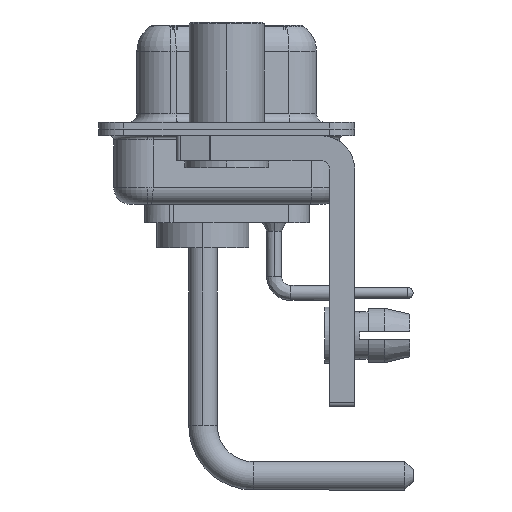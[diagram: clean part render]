
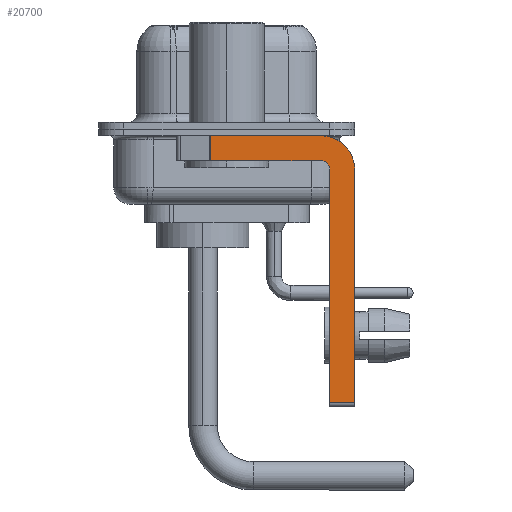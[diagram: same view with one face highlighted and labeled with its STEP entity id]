
A CAD part, left-side view. The second image highlights one B-rep face of the part: STEP entity #20700.
In plain terms, the highlighted planar face has unit normal (-1, 0, 0).
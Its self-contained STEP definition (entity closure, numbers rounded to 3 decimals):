
#186 = ORIENTED_EDGE ( 'NONE', *, *, #3425, .T. ) ;
#244 = VERTEX_POINT ( 'NONE', #5810 ) ;
#465 = VERTEX_POINT ( 'NONE', #19800 ) ;
#865 = LINE ( 'NONE', #9056, #3187 ) ;
#1306 = CARTESIAN_POINT ( 'NONE',  ( -2.9, -7.65, -2.4 ) ) ;
#1475 = CARTESIAN_POINT ( 'NONE',  ( -2.9, -5.65, -1.9 ) ) ;
#1550 = CARTESIAN_POINT ( 'NONE',  ( -2.9, -5.65, -1.9 ) ) ;
#1585 = AXIS2_PLACEMENT_3D ( 'NONE', #14145, #19778, #5796 ) ;
#1622 = DIRECTION ( 'NONE',  ( 1., 0., 0. ) ) ;
#2145 = VECTOR ( 'NONE', #5016, 1000. ) ;
#2606 = CARTESIAN_POINT ( 'NONE',  ( -2.9, -5.65, -2.4 ) ) ;
#2700 = LINE ( 'NONE', #22467, #2145 ) ;
#2841 = EDGE_CURVE ( 'NONE', #244, #4026, #12103, .T. ) ;
#2920 = CARTESIAN_POINT ( 'NONE',  ( -2.9, 3., -0.4 ) ) ;
#3058 = CARTESIAN_POINT ( 'NONE',  ( -2.9, -7.65, -2.4 ) ) ;
#3187 = VECTOR ( 'NONE', #5215, 1000. ) ;
#3425 = EDGE_CURVE ( 'NONE', #14927, #16375, #865, .T. ) ;
#4026 = VERTEX_POINT ( 'NONE', #23267 ) ;
#4551 = CARTESIAN_POINT ( 'NONE',  ( -2.9, -6.15, -2.4 ) ) ;
#5016 = DIRECTION ( 'NONE',  ( 0., 0., 1. ) ) ;
#5215 = DIRECTION ( 'NONE',  ( 0., 0., -1. ) ) ;
#5321 = VECTOR ( 'NONE', #22303, 1000. ) ;
#5400 = DIRECTION ( 'NONE',  ( 0., 0., -1. ) ) ;
#5796 = DIRECTION ( 'NONE',  ( 0., 0., 1. ) ) ;
#5810 = CARTESIAN_POINT ( 'NONE',  ( -2.9, -6.15, -16.35 ) ) ;
#6831 = ORIENTED_EDGE ( 'NONE', *, *, #7423, .F. ) ;
#6863 = ORIENTED_EDGE ( 'NONE', *, *, #2841, .T. ) ;
#6867 = VECTOR ( 'NONE', #23519, 1000. ) ;
#7423 = EDGE_CURVE ( 'NONE', #18078, #16375, #23031, .T. ) ;
#7521 = FACE_OUTER_BOUND ( 'NONE', #20593, .T. ) ;
#7648 = DIRECTION ( 'NONE',  ( 0., 0., -1. ) ) ;
#8011 = DIRECTION ( 'NONE',  ( 1., 0., 0. ) ) ;
#8805 = VECTOR ( 'NONE', #19782, 1000. ) ;
#9056 = CARTESIAN_POINT ( 'NONE',  ( -2.9, 0.978, -1.9 ) ) ;
#9861 = AXIS2_PLACEMENT_3D ( 'NONE', #13315, #1622, #7648 ) ;
#10473 = ORIENTED_EDGE ( 'NONE', *, *, #22078, .F. ) ;
#12103 = LINE ( 'NONE', #16083, #6867 ) ;
#12815 = ORIENTED_EDGE ( 'NONE', *, *, #14926, .F. ) ;
#13247 = LINE ( 'NONE', #1306, #14360 ) ;
#13315 = CARTESIAN_POINT ( 'NONE',  ( -2.9, -5.65, -2.4 ) ) ;
#13697 = ORIENTED_EDGE ( 'NONE', *, *, #19569, .F. ) ;
#14145 = CARTESIAN_POINT ( 'NONE',  ( -2.9, -5.65, -2.4 ) ) ;
#14195 = EDGE_CURVE ( 'NONE', #17536, #18078, #14717, .T. ) ;
#14360 = VECTOR ( 'NONE', #5400, 1000. ) ;
#14717 = CIRCLE ( 'NONE', #1585, 0.5 ) ;
#14926 = EDGE_CURVE ( 'NONE', #14927, #465, #20127, .T. ) ;
#14927 = VERTEX_POINT ( 'NONE', #18211 ) ;
#15280 = ORIENTED_EDGE ( 'NONE', *, *, #22847, .F. ) ;
#16083 = CARTESIAN_POINT ( 'NONE',  ( -2.9, -5.65, -16.35 ) ) ;
#16231 = DIRECTION ( 'NONE',  ( 0., 0., -1. ) ) ;
#16375 = VERTEX_POINT ( 'NONE', #18848 ) ;
#16972 = CIRCLE ( 'NONE', #23502, 2. ) ;
#17536 = VERTEX_POINT ( 'NONE', #4551 ) ;
#18078 = VERTEX_POINT ( 'NONE', #1550 ) ;
#18211 = CARTESIAN_POINT ( 'NONE',  ( -2.9, 0.978, -0.4 ) ) ;
#18272 = ORIENTED_EDGE ( 'NONE', *, *, #14195, .F. ) ;
#18848 = CARTESIAN_POINT ( 'NONE',  ( -2.9, 0.978, -1.9 ) ) ;
#19465 = PLANE ( 'NONE',  #9861 ) ;
#19569 = EDGE_CURVE ( 'NONE', #24074, #4026, #13247, .T. ) ;
#19778 = DIRECTION ( 'NONE',  ( -1., 0., 0. ) ) ;
#19782 = DIRECTION ( 'NONE',  ( 0., 1., 0. ) ) ;
#19800 = CARTESIAN_POINT ( 'NONE',  ( -2.9, -5.65, -0.4 ) ) ;
#20127 = LINE ( 'NONE', #2920, #5321 ) ;
#20593 = EDGE_LOOP ( 'NONE', ( #12815, #186, #6831, #18272, #10473, #6863, #13697, #15280 ) ) ;
#20700 = ADVANCED_FACE ( 'NONE', ( #7521 ), #19465, .F. ) ;
#22078 = EDGE_CURVE ( 'NONE', #244, #17536, #2700, .T. ) ;
#22303 = DIRECTION ( 'NONE',  ( 0., -1., 0. ) ) ;
#22467 = CARTESIAN_POINT ( 'NONE',  ( -2.9, -6.15, -16.6 ) ) ;
#22847 = EDGE_CURVE ( 'NONE', #465, #24074, #16972, .T. ) ;
#23031 = LINE ( 'NONE', #1475, #8805 ) ;
#23267 = CARTESIAN_POINT ( 'NONE',  ( -2.9, -7.65, -16.35 ) ) ;
#23502 = AXIS2_PLACEMENT_3D ( 'NONE', #2606, #8011, #16231 ) ;
#23519 = DIRECTION ( 'NONE',  ( 0., -1., 0. ) ) ;
#24074 = VERTEX_POINT ( 'NONE', #3058 ) ;
